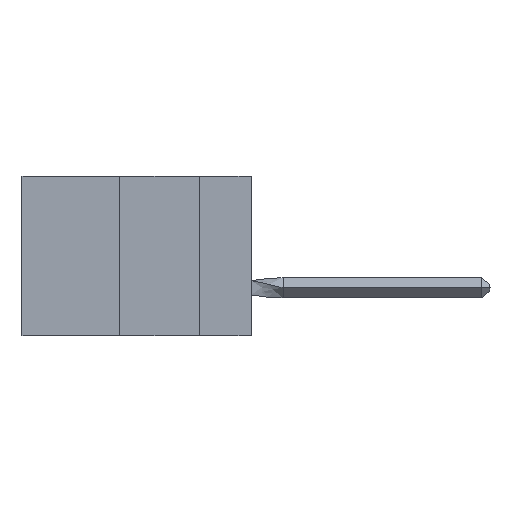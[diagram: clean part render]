
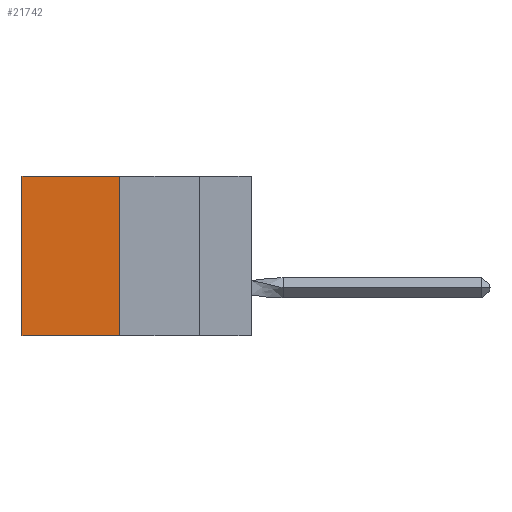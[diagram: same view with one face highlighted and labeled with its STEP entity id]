
A CAD part, left-side view. The second image highlights one B-rep face of the part: STEP entity #21742.
In plain terms, the highlighted planar face has unit normal (-1, 0, 0).
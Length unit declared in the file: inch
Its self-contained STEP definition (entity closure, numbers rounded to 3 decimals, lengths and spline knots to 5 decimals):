
#651 = CARTESIAN_POINT ( 'NONE',  ( 0.305, 0.72, -0.5 ) ) ;
#973 = VECTOR ( 'NONE', #19340, 39.37008 ) ;
#1513 = EDGE_CURVE ( 'NONE', #14930, #34241, #16409, .T. ) ;
#3022 = CARTESIAN_POINT ( 'NONE',  ( 0.305, 0.413, -0.5 ) ) ;
#3343 = LINE ( 'NONE', #34222, #973 ) ;
#3863 = CARTESIAN_POINT ( 'NONE',  ( 0.305, 0.413, 0. ) ) ;
#8216 = CARTESIAN_POINT ( 'NONE',  ( 0.305, 0.413, 0. ) ) ;
#10243 = VECTOR ( 'NONE', #22245, 39.37008 ) ;
#12108 = CARTESIAN_POINT ( 'NONE',  ( 0.305, 0.72, -0.5 ) ) ;
#14406 = PLANE ( 'NONE',  #18833 ) ;
#14521 = ORIENTED_EDGE ( 'NONE', *, *, #28319, .F. ) ;
#14930 = VERTEX_POINT ( 'NONE', #21973 ) ;
#15592 = ORIENTED_EDGE ( 'NONE', *, *, #31328, .T. ) ;
#16409 = LINE ( 'NONE', #28311, #10243 ) ;
#17341 = LINE ( 'NONE', #651, #27733 ) ;
#18030 = DIRECTION ( 'NONE',  ( 1., 0., 0. ) ) ;
#18833 = AXIS2_PLACEMENT_3D ( 'NONE', #3022, #18030, #24323 ) ;
#19340 = DIRECTION ( 'NONE',  ( 0., 0., -1. ) ) ;
#21742 = ADVANCED_FACE ( 'NONE', ( #30932 ), #14406, .F. ) ;
#21973 = CARTESIAN_POINT ( 'NONE',  ( 0.305, 0.413, -0.5 ) ) ;
#22245 = DIRECTION ( 'NONE',  ( 0., 1., 0. ) ) ;
#22371 = ORIENTED_EDGE ( 'NONE', *, *, #1513, .F. ) ;
#24323 = DIRECTION ( 'NONE',  ( 0., 0., -1. ) ) ;
#25253 = DIRECTION ( 'NONE',  ( 0., 0., -1. ) ) ;
#26035 = EDGE_CURVE ( 'NONE', #35091, #29903, #37048, .T. ) ;
#27733 = VECTOR ( 'NONE', #25253, 39.37008 ) ;
#28104 = DIRECTION ( 'NONE',  ( 0., 1., 0. ) ) ;
#28311 = CARTESIAN_POINT ( 'NONE',  ( 0.305, 0.413, -0.5 ) ) ;
#28319 = EDGE_CURVE ( 'NONE', #35091, #14930, #3343, .T. ) ;
#29525 = VECTOR ( 'NONE', #28104, 39.37008 ) ;
#29903 = VERTEX_POINT ( 'NONE', #36780 ) ;
#30650 = EDGE_LOOP ( 'NONE', ( #15592, #22371, #14521, #34385 ) ) ;
#30932 = FACE_OUTER_BOUND ( 'NONE', #30650, .T. ) ;
#31328 = EDGE_CURVE ( 'NONE', #29903, #34241, #17341, .T. ) ;
#34222 = CARTESIAN_POINT ( 'NONE',  ( 0.305, 0.413, -0.5 ) ) ;
#34241 = VERTEX_POINT ( 'NONE', #12108 ) ;
#34385 = ORIENTED_EDGE ( 'NONE', *, *, #26035, .T. ) ;
#35091 = VERTEX_POINT ( 'NONE', #8216 ) ;
#36780 = CARTESIAN_POINT ( 'NONE',  ( 0.305, 0.72, 0. ) ) ;
#37048 = LINE ( 'NONE', #3863, #29525 ) ;
